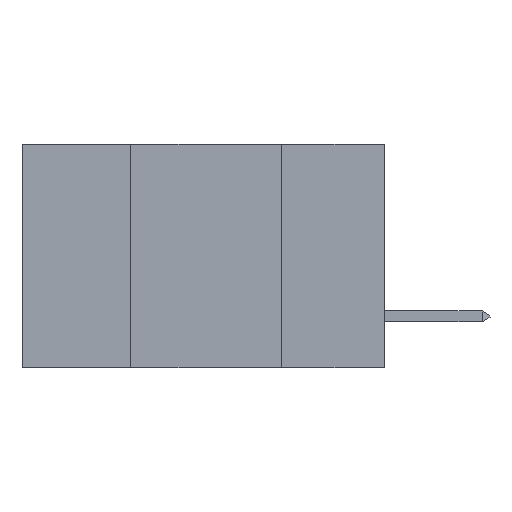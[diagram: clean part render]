
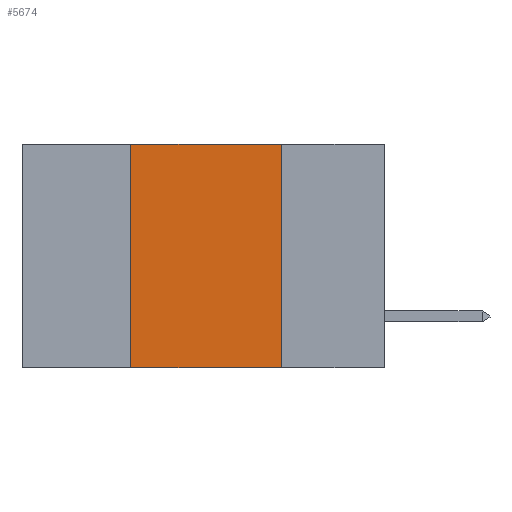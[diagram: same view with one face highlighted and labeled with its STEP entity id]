
A CAD part, left-side view. The second image highlights one B-rep face of the part: STEP entity #5674.
In plain terms, the highlighted planar face has unit normal (-1, 0, 0).
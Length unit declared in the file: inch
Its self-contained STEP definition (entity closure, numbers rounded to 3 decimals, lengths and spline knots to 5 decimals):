
#1082 = ORIENTED_EDGE ( 'NONE', *, *, #7732, .F. ) ;
#1108 = VECTOR ( 'NONE', #1451, 39.37008 ) ;
#1246 = ORIENTED_EDGE ( 'NONE', *, *, #3374, .F. ) ;
#1451 = DIRECTION ( 'NONE',  ( 0., -1., 0. ) ) ;
#2287 = CARTESIAN_POINT ( 'NONE',  ( 0., 0.6, 0. ) ) ;
#3374 = EDGE_CURVE ( 'NONE', #18828, #4924, #10674, .T. ) ;
#4820 = VERTEX_POINT ( 'NONE', #17865 ) ;
#4924 = VERTEX_POINT ( 'NONE', #12887 ) ;
#5674 = ADVANCED_FACE ( 'NONE', ( #9835 ), #16566, .F. ) ;
#6847 = CARTESIAN_POINT ( 'NONE',  ( 0., 0.6, 0. ) ) ;
#6949 = CARTESIAN_POINT ( 'NONE',  ( 0., 0.42, -0.37 ) ) ;
#7732 = EDGE_CURVE ( 'NONE', #17758, #18828, #18082, .T. ) ;
#7765 = DIRECTION ( 'NONE',  ( 1., 0., 0. ) ) ;
#7831 = LINE ( 'NONE', #11359, #21319 ) ;
#8962 = ORIENTED_EDGE ( 'NONE', *, *, #15264, .T. ) ;
#9835 = FACE_OUTER_BOUND ( 'NONE', #12412, .T. ) ;
#9920 = CARTESIAN_POINT ( 'NONE',  ( 0., 0.42, 0. ) ) ;
#10674 = LINE ( 'NONE', #6847, #1108 ) ;
#11122 = VECTOR ( 'NONE', #12132, 39.37008 ) ;
#11359 = CARTESIAN_POINT ( 'NONE',  ( 0., 0.17, 0. ) ) ;
#12132 = DIRECTION ( 'NONE',  ( 0., -1., 0. ) ) ;
#12412 = EDGE_LOOP ( 'NONE', ( #15377, #1246, #1082, #8962 ) ) ;
#12887 = CARTESIAN_POINT ( 'NONE',  ( 0., 0.17, 0. ) ) ;
#13169 = AXIS2_PLACEMENT_3D ( 'NONE', #2287, #7765, #20088 ) ;
#15264 = EDGE_CURVE ( 'NONE', #17758, #4820, #15832, .T. ) ;
#15377 = ORIENTED_EDGE ( 'NONE', *, *, #19956, .F. ) ;
#15832 = LINE ( 'NONE', #20909, #11122 ) ;
#16566 = PLANE ( 'NONE',  #13169 ) ;
#17261 = CARTESIAN_POINT ( 'NONE',  ( 0., 0.42, 0. ) ) ;
#17532 = VECTOR ( 'NONE', #20770, 39.37008 ) ;
#17758 = VERTEX_POINT ( 'NONE', #6949 ) ;
#17865 = CARTESIAN_POINT ( 'NONE',  ( 0., 0.17, -0.37 ) ) ;
#18082 = LINE ( 'NONE', #17261, #17532 ) ;
#18828 = VERTEX_POINT ( 'NONE', #9920 ) ;
#19956 = EDGE_CURVE ( 'NONE', #4924, #4820, #7831, .T. ) ;
#20088 = DIRECTION ( 'NONE',  ( 0., 0., -1. ) ) ;
#20150 = DIRECTION ( 'NONE',  ( 0., 0., -1. ) ) ;
#20770 = DIRECTION ( 'NONE',  ( 0., 0., 1. ) ) ;
#20909 = CARTESIAN_POINT ( 'NONE',  ( 0., 0.6, -0.37 ) ) ;
#21319 = VECTOR ( 'NONE', #20150, 39.37008 ) ;
